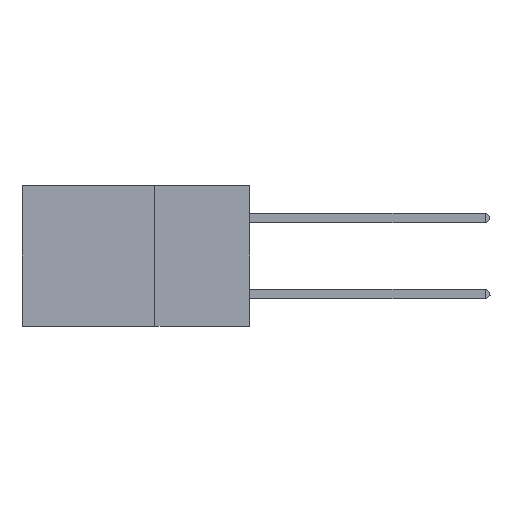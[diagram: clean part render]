
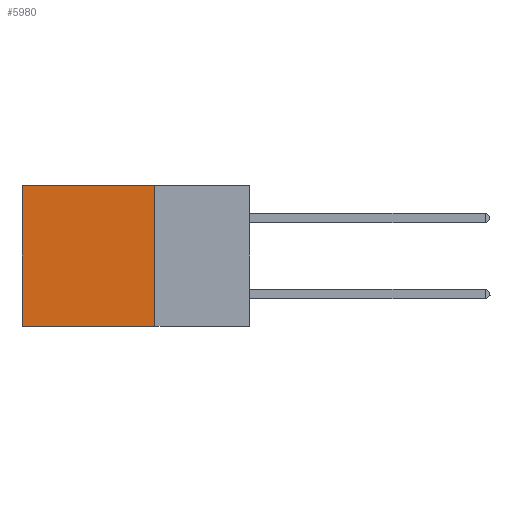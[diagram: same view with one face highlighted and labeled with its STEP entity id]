
A CAD part, left-side view. The second image highlights one B-rep face of the part: STEP entity #5980.
In plain terms, the highlighted planar face has unit normal (-1, 0, 0).
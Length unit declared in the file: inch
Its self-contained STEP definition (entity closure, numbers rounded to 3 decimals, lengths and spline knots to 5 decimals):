
#425 = CARTESIAN_POINT ( 'NONE',  ( 0.2875, 0.25, 0. ) ) ;
#593 = ORIENTED_EDGE ( 'NONE', *, *, #24042, .F. ) ;
#1633 = ORIENTED_EDGE ( 'NONE', *, *, #23958, .F. ) ;
#1893 = CARTESIAN_POINT ( 'NONE',  ( 0.2875, 0.25, -0.37 ) ) ;
#2153 = CARTESIAN_POINT ( 'NONE',  ( 0.2875, 0.25, 0. ) ) ;
#2520 = CARTESIAN_POINT ( 'NONE',  ( 0.2875, 0.25, 0. ) ) ;
#2818 = LINE ( 'NONE', #17199, #6703 ) ;
#3140 = EDGE_CURVE ( 'NONE', #7368, #11117, #10592, .T. ) ;
#4137 = DIRECTION ( 'NONE',  ( 0., 0., -1. ) ) ;
#4143 = AXIS2_PLACEMENT_3D ( 'NONE', #25737, #23699, #13255 ) ;
#4680 = DIRECTION ( 'NONE',  ( 0., 0., -1. ) ) ;
#5198 = PLANE ( 'NONE',  #4143 ) ;
#5721 = LINE ( 'NONE', #2520, #24598 ) ;
#5980 = ADVANCED_FACE ( 'NONE', ( #12967 ), #5198, .F. ) ;
#6510 = VERTEX_POINT ( 'NONE', #23418 ) ;
#6589 = ORIENTED_EDGE ( 'NONE', *, *, #3140, .T. ) ;
#6703 = VECTOR ( 'NONE', #11007, 39.37008 ) ;
#7325 = VERTEX_POINT ( 'NONE', #1893 ) ;
#7368 = VERTEX_POINT ( 'NONE', #2153 ) ;
#7937 = LINE ( 'NONE', #12454, #23019 ) ;
#10592 = LINE ( 'NONE', #425, #17951 ) ;
#11007 = DIRECTION ( 'NONE',  ( 0., 1., 0. ) ) ;
#11117 = VERTEX_POINT ( 'NONE', #20953 ) ;
#12454 = CARTESIAN_POINT ( 'NONE',  ( 0.2875, 0.6, 0. ) ) ;
#12967 = FACE_OUTER_BOUND ( 'NONE', #26001, .T. ) ;
#13255 = DIRECTION ( 'NONE',  ( 0., 0., -1. ) ) ;
#13636 = EDGE_CURVE ( 'NONE', #11117, #6510, #7937, .T. ) ;
#17199 = CARTESIAN_POINT ( 'NONE',  ( 0.2875, 0.25, -0.37 ) ) ;
#17951 = VECTOR ( 'NONE', #25174, 39.37008 ) ;
#19362 = ORIENTED_EDGE ( 'NONE', *, *, #13636, .T. ) ;
#20953 = CARTESIAN_POINT ( 'NONE',  ( 0.2875, 0.6, 0. ) ) ;
#23019 = VECTOR ( 'NONE', #4137, 39.37008 ) ;
#23418 = CARTESIAN_POINT ( 'NONE',  ( 0.2875, 0.6, -0.37 ) ) ;
#23699 = DIRECTION ( 'NONE',  ( 1., 0., 0. ) ) ;
#23958 = EDGE_CURVE ( 'NONE', #7325, #6510, #2818, .T. ) ;
#24042 = EDGE_CURVE ( 'NONE', #7368, #7325, #5721, .T. ) ;
#24598 = VECTOR ( 'NONE', #4680, 39.37008 ) ;
#25174 = DIRECTION ( 'NONE',  ( 0., 1., 0. ) ) ;
#25737 = CARTESIAN_POINT ( 'NONE',  ( 0.2875, 0.25, 0. ) ) ;
#26001 = EDGE_LOOP ( 'NONE', ( #19362, #1633, #593, #6589 ) ) ;
